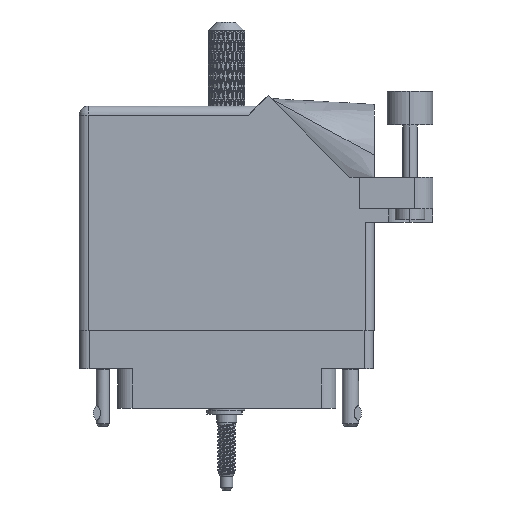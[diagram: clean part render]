
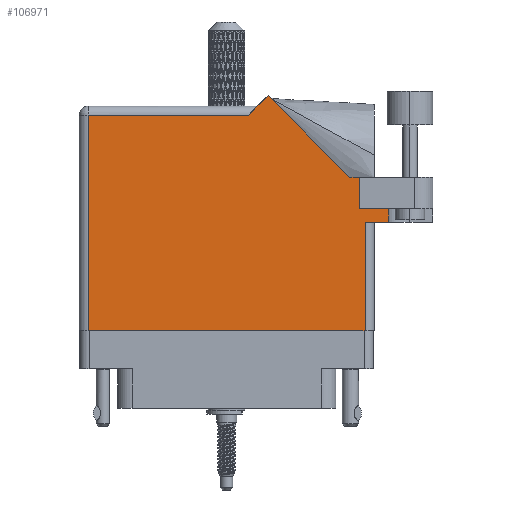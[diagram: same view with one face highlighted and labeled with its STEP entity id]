
A CAD part, front view. The second image highlights one B-rep face of the part: STEP entity #106971.
In plain terms, the highlighted face is planar.
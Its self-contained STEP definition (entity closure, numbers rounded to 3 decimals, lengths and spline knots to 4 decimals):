
#240 = ORIENTED_EDGE ( 'NONE', *, *, #37026, .T. ) ;
#6008 = VERTEX_POINT ( 'NONE', #39215 ) ;
#7575 = EDGE_CURVE ( 'NONE', #46881, #37743, #37072, .T. ) ;
#11634 = CARTESIAN_POINT ( 'NONE',  ( 2.1115, 0.737, 0. ) ) ;
#12731 = VERTEX_POINT ( 'NONE', #36770 ) ;
#12784 = VERTEX_POINT ( 'NONE', #29014 ) ;
#13088 = VECTOR ( 'NONE', #56611, 39.3701 ) ;
#13137 = DIRECTION ( 'NONE',  ( 0., 1., 0. ) ) ;
#14555 = ORIENTED_EDGE ( 'NONE', *, *, #84938, .T. ) ;
#14976 = DIRECTION ( 'NONE',  ( 1., 0., 0. ) ) ;
#17095 = EDGE_CURVE ( 'NONE', #12784, #20462, #97691, .T. ) ;
#18048 = CARTESIAN_POINT ( 'NONE',  ( 0.062, 0., 0. ) ) ;
#19334 = EDGE_CURVE ( 'NONE', #62187, #46881, #80770, .T. ) ;
#20120 = LINE ( 'NONE', #23217, #42067 ) ;
#20354 = AXIS2_PLACEMENT_3D ( 'NONE', #105937, #96695, #105556 ) ;
#20462 = VERTEX_POINT ( 'NONE', #93256 ) ;
#21212 = DIRECTION ( 'NONE',  ( 1., 0., 0. ) ) ;
#21946 = ORIENTED_EDGE ( 'NONE', *, *, #19334, .T. ) ;
#21984 = CARTESIAN_POINT ( 'NONE',  ( 1.91, 0.831, 0. ) ) ;
#22627 = LINE ( 'NONE', #21984, #72332 ) ;
#22753 = CARTESIAN_POINT ( 'NONE',  ( 1.8444, 1.044, 0. ) ) ;
#23217 = CARTESIAN_POINT ( 'NONE',  ( 1.217, 1.53, 0. ) ) ;
#23429 = CARTESIAN_POINT ( 'NONE',  ( 0., 0., 0. ) ) ;
#23770 = CARTESIAN_POINT ( 'NONE',  ( 1.948, 0., 0. ) ) ;
#24469 = EDGE_CURVE ( 'NONE', #6008, #103379, #20120, .T. ) ;
#25398 = LINE ( 'NONE', #22753, #48817 ) ;
#27026 = CARTESIAN_POINT ( 'NONE',  ( 1.155, 1.468, 0. ) ) ;
#27034 = ORIENTED_EDGE ( 'NONE', *, *, #46238, .T. ) ;
#28205 = CARTESIAN_POINT ( 'NONE',  ( 1.948, 0.737, 0. ) ) ;
#29014 = CARTESIAN_POINT ( 'NONE',  ( 1.91, 1.044, 0. ) ) ;
#29975 = CARTESIAN_POINT ( 'NONE',  ( 0.062, 0., 0. ) ) ;
#31999 = EDGE_CURVE ( 'NONE', #103379, #12731, #41199, .T. ) ;
#32712 = DIRECTION ( 'NONE',  ( -1., 0., 0. ) ) ;
#35831 = ORIENTED_EDGE ( 'NONE', *, *, #7575, .T. ) ;
#36770 = CARTESIAN_POINT ( 'NONE',  ( 0.062, 1.468, 0. ) ) ;
#37026 = EDGE_CURVE ( 'NONE', #98040, #62187, #81268, .T. ) ;
#37072 = LINE ( 'NONE', #110996, #50891 ) ;
#37743 = VERTEX_POINT ( 'NONE', #11634 ) ;
#38244 = ORIENTED_EDGE ( 'NONE', *, *, #60765, .F. ) ;
#38688 = ORIENTED_EDGE ( 'NONE', *, *, #31999, .T. ) ;
#39215 = CARTESIAN_POINT ( 'NONE',  ( 1.2877, 1.6007, 0. ) ) ;
#39782 = VECTOR ( 'NONE', #32712, 39.3701 ) ;
#41199 = LINE ( 'NONE', #103682, #39782 ) ;
#42067 = VECTOR ( 'NONE', #84918, 39.3701 ) ;
#44976 = PLANE ( 'NONE',  #20354 ) ;
#46202 = CARTESIAN_POINT ( 'NONE',  ( 1.91, 0.831, 0. ) ) ;
#46225 = EDGE_CURVE ( 'NONE', #20462, #6008, #25398, .T. ) ;
#46238 = EDGE_CURVE ( 'NONE', #106189, #12784, #22627, .T. ) ;
#46881 = VERTEX_POINT ( 'NONE', #56810 ) ;
#48817 = VECTOR ( 'NONE', #75185, 39.3701 ) ;
#49275 = VECTOR ( 'NONE', #69121, 39.3701 ) ;
#50891 = VECTOR ( 'NONE', #21212, 39.3701 ) ;
#51314 = CARTESIAN_POINT ( 'NONE',  ( 2.41, 1.044, 0. ) ) ;
#52965 = CARTESIAN_POINT ( 'NONE',  ( 2.1115, 0.831, 0. ) ) ;
#53406 = DIRECTION ( 'NONE',  ( 0., -1., 0. ) ) ;
#56371 = EDGE_CURVE ( 'NONE', #83270, #37743, #63993, .T. ) ;
#56611 = DIRECTION ( 'NONE',  ( 0., -1., 0. ) ) ;
#56810 = CARTESIAN_POINT ( 'NONE',  ( 1.948, 0.737, 0. ) ) ;
#59110 = VECTOR ( 'NONE', #14976, 39.3701 ) ;
#60765 = EDGE_CURVE ( 'NONE', #106189, #83270, #85332, .T. ) ;
#62187 = VERTEX_POINT ( 'NONE', #23770 ) ;
#63993 = LINE ( 'NONE', #88946, #70923 ) ;
#64393 = DIRECTION ( 'NONE',  ( 1., 0., 0. ) ) ;
#69121 = DIRECTION ( 'NONE',  ( -1., 0., 0. ) ) ;
#70923 = VECTOR ( 'NONE', #53406, 39.3701 ) ;
#72332 = VECTOR ( 'NONE', #13137, 39.3701 ) ;
#75185 = DIRECTION ( 'NONE',  ( -0.707, 0.707, 0. ) ) ;
#77352 = ORIENTED_EDGE ( 'NONE', *, *, #46225, .T. ) ;
#80770 = LINE ( 'NONE', #28205, #95944 ) ;
#81268 = LINE ( 'NONE', #23429, #59110 ) ;
#83270 = VERTEX_POINT ( 'NONE', #52965 ) ;
#83282 = FACE_OUTER_BOUND ( 'NONE', #99940, .T. ) ;
#84918 = DIRECTION ( 'NONE',  ( -0.707, -0.707, 0. ) ) ;
#84938 = EDGE_CURVE ( 'NONE', #12731, #98040, #87588, .T. ) ;
#85332 = LINE ( 'NONE', #91739, #107492 ) ;
#86986 = ORIENTED_EDGE ( 'NONE', *, *, #17095, .T. ) ;
#87588 = LINE ( 'NONE', #29975, #13088 ) ;
#88946 = CARTESIAN_POINT ( 'NONE',  ( 2.1115, 1.1618, 0. ) ) ;
#89210 = DIRECTION ( 'NONE',  ( 0., 1., 0. ) ) ;
#91739 = CARTESIAN_POINT ( 'NONE',  ( 1.91, 0.831, 0. ) ) ;
#93256 = CARTESIAN_POINT ( 'NONE',  ( 1.8444, 1.044, 0. ) ) ;
#95280 = ORIENTED_EDGE ( 'NONE', *, *, #56371, .F. ) ;
#95944 = VECTOR ( 'NONE', #89210, 39.3701 ) ;
#96695 = DIRECTION ( 'NONE',  ( 0., 0., -1. ) ) ;
#97691 = LINE ( 'NONE', #51314, #49275 ) ;
#98040 = VERTEX_POINT ( 'NONE', #18048 ) ;
#99940 = EDGE_LOOP ( 'NONE', ( #240, #21946, #35831, #95280, #38244, #27034, #86986, #77352, #102573, #38688, #14555 ) ) ;
#102573 = ORIENTED_EDGE ( 'NONE', *, *, #24469, .T. ) ;
#103379 = VERTEX_POINT ( 'NONE', #27026 ) ;
#103682 = CARTESIAN_POINT ( 'NONE',  ( 0., 1.468, 0. ) ) ;
#105556 = DIRECTION ( 'NONE',  ( -1., 0., 0. ) ) ;
#105937 = CARTESIAN_POINT ( 'NONE',  ( 0., 1.53, 0. ) ) ;
#106189 = VERTEX_POINT ( 'NONE', #46202 ) ;
#106971 = ADVANCED_FACE ( 'NONE', ( #83282 ), #44976, .F. ) ;
#107492 = VECTOR ( 'NONE', #64393, 39.3701 ) ;
#110996 = CARTESIAN_POINT ( 'NONE',  ( 2.01, 0.737, 0. ) ) ;
